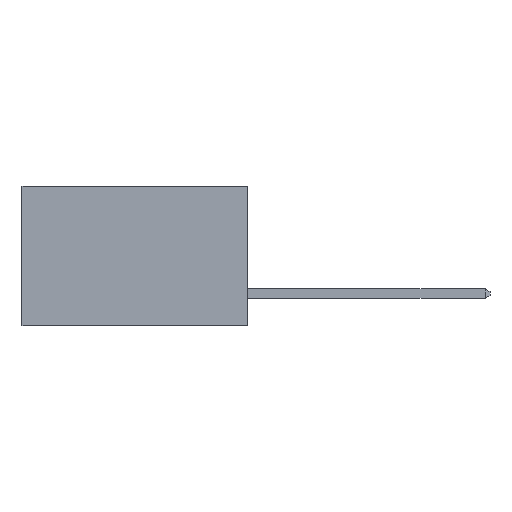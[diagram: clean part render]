
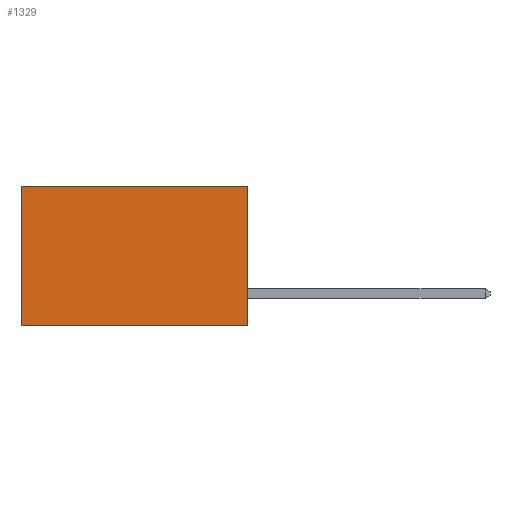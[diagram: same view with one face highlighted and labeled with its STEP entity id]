
A CAD part, left-side view. The second image highlights one B-rep face of the part: STEP entity #1329.
In plain terms, the highlighted planar face has unit normal (-1, 0, 0).
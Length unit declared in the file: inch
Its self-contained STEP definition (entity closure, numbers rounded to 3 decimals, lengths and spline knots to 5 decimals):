
#610 = VERTEX_POINT ( 'NONE', #10009 ) ;
#906 = VECTOR ( 'NONE', #10370, 39.37008 ) ;
#1329 = ADVANCED_FACE ( 'NONE', ( #10245 ), #9290, .F. ) ;
#1334 = EDGE_CURVE ( 'NONE', #10206, #6014, #5797, .T. ) ;
#1364 = EDGE_CURVE ( 'NONE', #610, #9932, #9983, .T. ) ;
#1701 = ORIENTED_EDGE ( 'NONE', *, *, #1364, .F. ) ;
#1837 = VECTOR ( 'NONE', #6469, 39.37008 ) ;
#2580 = EDGE_LOOP ( 'NONE', ( #7284, #1701, #9994, #10756 ) ) ;
#3237 = LINE ( 'NONE', #9236, #906 ) ;
#3323 = VECTOR ( 'NONE', #7462, 39.37008 ) ;
#4149 = AXIS2_PLACEMENT_3D ( 'NONE', #8597, #7977, #6987 ) ;
#4747 = EDGE_CURVE ( 'NONE', #10206, #610, #7734, .T. ) ;
#5466 = EDGE_CURVE ( 'NONE', #6014, #9932, #3237, .T. ) ;
#5552 = CARTESIAN_POINT ( 'NONE',  ( 0.2615, 0., -0.37 ) ) ;
#5797 = LINE ( 'NONE', #7935, #1837 ) ;
#6014 = VERTEX_POINT ( 'NONE', #8845 ) ;
#6469 = DIRECTION ( 'NONE',  ( 0., 1., 0. ) ) ;
#6768 = CARTESIAN_POINT ( 'NONE',  ( 0.2615, 0., 0. ) ) ;
#6987 = DIRECTION ( 'NONE',  ( 0., 0., -1. ) ) ;
#7284 = ORIENTED_EDGE ( 'NONE', *, *, #5466, .T. ) ;
#7462 = DIRECTION ( 'NONE',  ( 0., 1., 0. ) ) ;
#7734 = LINE ( 'NONE', #10416, #7975 ) ;
#7935 = CARTESIAN_POINT ( 'NONE',  ( 0.2615, 0., 0. ) ) ;
#7975 = VECTOR ( 'NONE', #10306, 39.37008 ) ;
#7977 = DIRECTION ( 'NONE',  ( 1., 0., 0. ) ) ;
#8597 = CARTESIAN_POINT ( 'NONE',  ( 0.2615, 0., -0.37 ) ) ;
#8845 = CARTESIAN_POINT ( 'NONE',  ( 0.2615, 0.6, 0. ) ) ;
#9236 = CARTESIAN_POINT ( 'NONE',  ( 0.2615, 0.6, -0.37 ) ) ;
#9290 = PLANE ( 'NONE',  #4149 ) ;
#9591 = CARTESIAN_POINT ( 'NONE',  ( 0.2615, 0.6, -0.37 ) ) ;
#9932 = VERTEX_POINT ( 'NONE', #9591 ) ;
#9983 = LINE ( 'NONE', #5552, #3323 ) ;
#9994 = ORIENTED_EDGE ( 'NONE', *, *, #4747, .F. ) ;
#10009 = CARTESIAN_POINT ( 'NONE',  ( 0.2615, 0., -0.37 ) ) ;
#10206 = VERTEX_POINT ( 'NONE', #6768 ) ;
#10245 = FACE_OUTER_BOUND ( 'NONE', #2580, .T. ) ;
#10306 = DIRECTION ( 'NONE',  ( 0., 0., -1. ) ) ;
#10370 = DIRECTION ( 'NONE',  ( 0., 0., -1. ) ) ;
#10416 = CARTESIAN_POINT ( 'NONE',  ( 0.2615, 0., -0.37 ) ) ;
#10756 = ORIENTED_EDGE ( 'NONE', *, *, #1334, .T. ) ;
